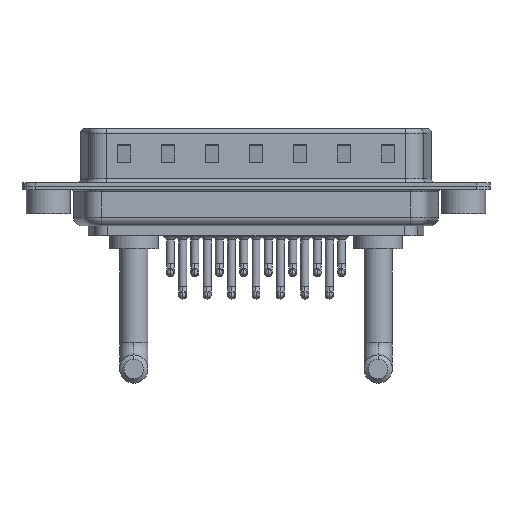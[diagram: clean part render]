
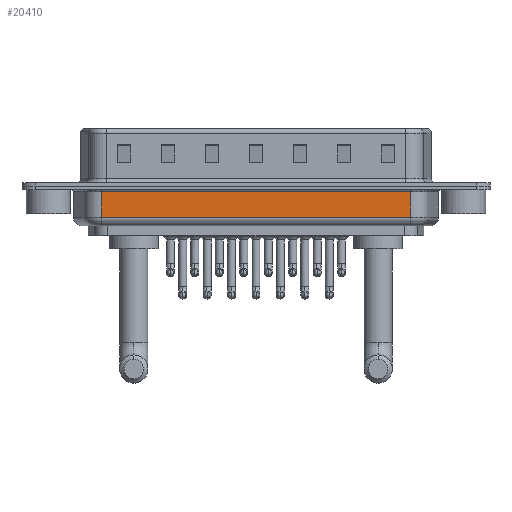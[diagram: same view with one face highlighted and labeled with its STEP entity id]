
A CAD part, front view. The second image highlights one B-rep face of the part: STEP entity #20410.
In plain terms, the highlighted planar face has unit normal (0, -1, 0).
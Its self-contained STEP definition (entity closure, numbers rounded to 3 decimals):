
#436 = EDGE_LOOP ( 'NONE', ( #1477, #11826, #1225, #11231 ) ) ;
#1225 = ORIENTED_EDGE ( 'NONE', *, *, #16446, .T. ) ;
#1477 = ORIENTED_EDGE ( 'NONE', *, *, #3836, .F. ) ;
#1555 = PLANE ( 'NONE',  #4257 ) ;
#3836 = EDGE_CURVE ( 'NONE', #4178, #10853, #11102, .T. ) ;
#4178 = VERTEX_POINT ( 'NONE', #14452 ) ;
#4257 = AXIS2_PLACEMENT_3D ( 'NONE', #24478, #5320, #4940 ) ;
#4940 = DIRECTION ( 'NONE',  ( 0., 0., 1. ) ) ;
#5076 = LINE ( 'NONE', #20711, #11060 ) ;
#5320 = DIRECTION ( 'NONE',  ( 0., 1., 0. ) ) ;
#5350 = CARTESIAN_POINT ( 'NONE',  ( 41.044, -5.35, -3.5 ) ) ;
#5770 = VECTOR ( 'NONE', #7464, 1000. ) ;
#6202 = VECTOR ( 'NONE', #18736, 1000. ) ;
#6479 = DIRECTION ( 'NONE',  ( 0., 0., 1. ) ) ;
#7218 = CARTESIAN_POINT ( 'NONE',  ( 6.006, -5.35, -4.5 ) ) ;
#7309 = DIRECTION ( 'NONE',  ( -1., 0., 0. ) ) ;
#7464 = DIRECTION ( 'NONE',  ( 1., 0., 0. ) ) ;
#7630 = CARTESIAN_POINT ( 'NONE',  ( 41.044, -5.35, -0.65 ) ) ;
#10545 = VECTOR ( 'NONE', #6479, 1000. ) ;
#10853 = VERTEX_POINT ( 'NONE', #19580 ) ;
#11060 = VECTOR ( 'NONE', #7309, 1000. ) ;
#11102 = LINE ( 'NONE', #7218, #6202 ) ;
#11231 = ORIENTED_EDGE ( 'NONE', *, *, #20343, .T. ) ;
#11826 = ORIENTED_EDGE ( 'NONE', *, *, #16721, .T. ) ;
#13751 = CARTESIAN_POINT ( 'NONE',  ( 41.044, -5.35, -4.5 ) ) ;
#14452 = CARTESIAN_POINT ( 'NONE',  ( 6.006, -5.35, -3.5 ) ) ;
#14777 = VERTEX_POINT ( 'NONE', #7630 ) ;
#16446 = EDGE_CURVE ( 'NONE', #16567, #14777, #23630, .T. ) ;
#16567 = VERTEX_POINT ( 'NONE', #5350 ) ;
#16721 = EDGE_CURVE ( 'NONE', #4178, #16567, #24637, .T. ) ;
#18736 = DIRECTION ( 'NONE',  ( 0., 0., 1. ) ) ;
#19580 = CARTESIAN_POINT ( 'NONE',  ( 6.006, -5.35, -0.65 ) ) ;
#20343 = EDGE_CURVE ( 'NONE', #14777, #10853, #5076, .T. ) ;
#20410 = ADVANCED_FACE ( 'NONE', ( #24351 ), #1555, .F. ) ;
#20711 = CARTESIAN_POINT ( 'NONE',  ( 6.006, -5.35, -0.65 ) ) ;
#21100 = CARTESIAN_POINT ( 'NONE',  ( 6.006, -5.35, -3.5 ) ) ;
#23630 = LINE ( 'NONE', #13751, #10545 ) ;
#24351 = FACE_OUTER_BOUND ( 'NONE', #436, .T. ) ;
#24478 = CARTESIAN_POINT ( 'NONE',  ( 6.006, -5.35, -4.5 ) ) ;
#24637 = LINE ( 'NONE', #21100, #5770 ) ;
